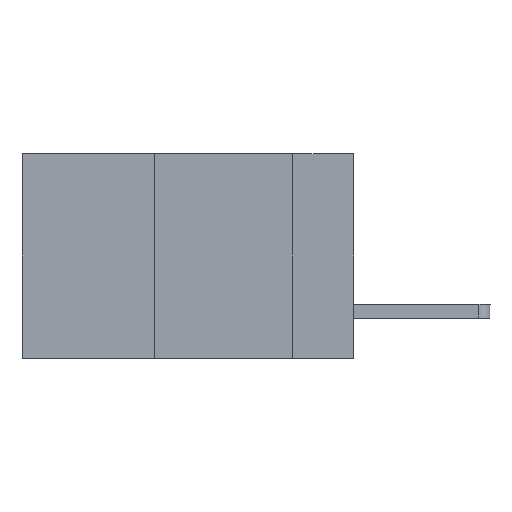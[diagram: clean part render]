
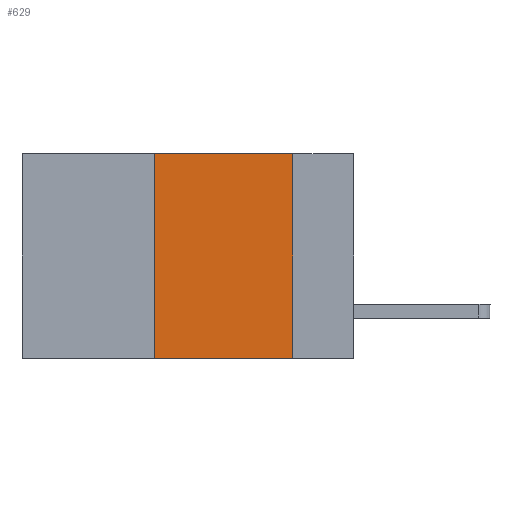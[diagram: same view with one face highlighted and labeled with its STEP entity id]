
A CAD part, left-side view. The second image highlights one B-rep face of the part: STEP entity #629.
In plain terms, the highlighted planar face has unit normal (-1, 0, 0).
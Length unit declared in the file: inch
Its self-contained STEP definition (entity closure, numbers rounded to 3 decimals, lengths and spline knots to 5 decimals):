
#412 = PLANE ( 'NONE',  #4542 ) ;
#437 = VERTEX_POINT ( 'NONE', #9485 ) ;
#629 = ADVANCED_FACE ( 'NONE', ( #7861 ), #412, .F. ) ;
#946 = CARTESIAN_POINT ( 'NONE',  ( 0., 0.36, -0.37 ) ) ;
#1518 = LINE ( 'NONE', #9852, #5155 ) ;
#1609 = ORIENTED_EDGE ( 'NONE', *, *, #3841, .F. ) ;
#1911 = DIRECTION ( 'NONE',  ( 0., 0., -1. ) ) ;
#1983 = VERTEX_POINT ( 'NONE', #946 ) ;
#2784 = CARTESIAN_POINT ( 'NONE',  ( 0., 0.6, 0. ) ) ;
#3841 = EDGE_CURVE ( 'NONE', #1983, #437, #5960, .T. ) ;
#4064 = LINE ( 'NONE', #2784, #4915 ) ;
#4162 = CARTESIAN_POINT ( 'NONE',  ( 0., 0.6, 0. ) ) ;
#4392 = VECTOR ( 'NONE', #7723, 39.37008 ) ;
#4519 = ORIENTED_EDGE ( 'NONE', *, *, #8756, .T. ) ;
#4542 = AXIS2_PLACEMENT_3D ( 'NONE', #4162, #6483, #1911 ) ;
#4915 = VECTOR ( 'NONE', #8164, 39.37008 ) ;
#5155 = VECTOR ( 'NONE', #8261, 39.37008 ) ;
#5228 = ORIENTED_EDGE ( 'NONE', *, *, #8666, .F. ) ;
#5384 = CARTESIAN_POINT ( 'NONE',  ( 0., 0.11, -0.37 ) ) ;
#5960 = LINE ( 'NONE', #7011, #4392 ) ;
#6420 = CARTESIAN_POINT ( 'NONE',  ( 0., 0.11, 0. ) ) ;
#6483 = DIRECTION ( 'NONE',  ( 1., 0., 0. ) ) ;
#6975 = LINE ( 'NONE', #6420, #7705 ) ;
#7011 = CARTESIAN_POINT ( 'NONE',  ( 0., 0.36, 0. ) ) ;
#7532 = CARTESIAN_POINT ( 'NONE',  ( 0., 0.11, 0. ) ) ;
#7705 = VECTOR ( 'NONE', #8717, 39.37008 ) ;
#7723 = DIRECTION ( 'NONE',  ( 0., 0., 1. ) ) ;
#7757 = ORIENTED_EDGE ( 'NONE', *, *, #9637, .F. ) ;
#7861 = FACE_OUTER_BOUND ( 'NONE', #8536, .T. ) ;
#8164 = DIRECTION ( 'NONE',  ( 0., -1., 0. ) ) ;
#8261 = DIRECTION ( 'NONE',  ( 0., -1., 0. ) ) ;
#8536 = EDGE_LOOP ( 'NONE', ( #7757, #5228, #1609, #4519 ) ) ;
#8666 = EDGE_CURVE ( 'NONE', #437, #9366, #4064, .T. ) ;
#8717 = DIRECTION ( 'NONE',  ( 0., 0., -1. ) ) ;
#8756 = EDGE_CURVE ( 'NONE', #1983, #9481, #1518, .T. ) ;
#9366 = VERTEX_POINT ( 'NONE', #7532 ) ;
#9481 = VERTEX_POINT ( 'NONE', #5384 ) ;
#9485 = CARTESIAN_POINT ( 'NONE',  ( 0., 0.36, 0. ) ) ;
#9637 = EDGE_CURVE ( 'NONE', #9366, #9481, #6975, .T. ) ;
#9852 = CARTESIAN_POINT ( 'NONE',  ( 0., 0.6, -0.37 ) ) ;
